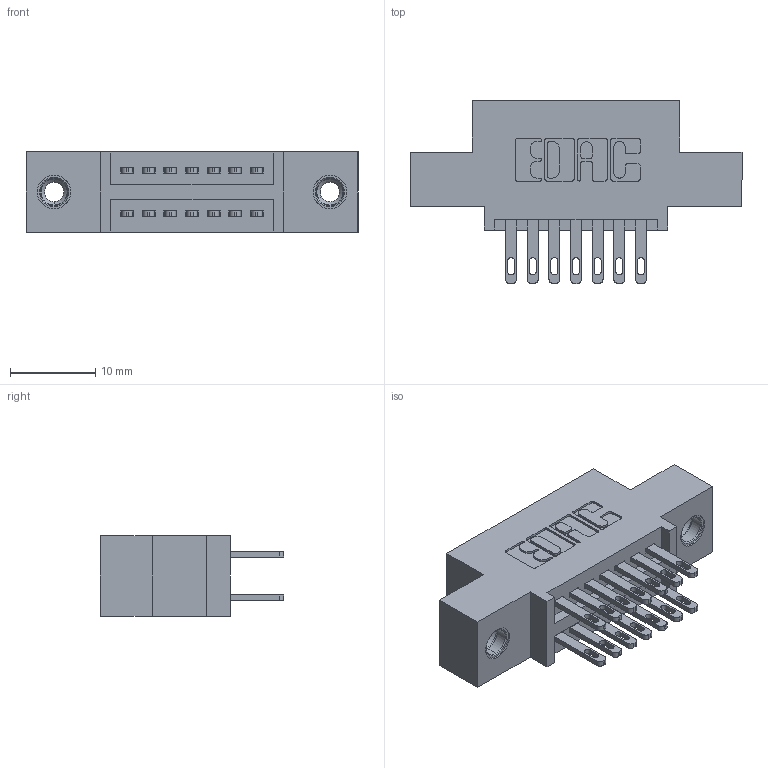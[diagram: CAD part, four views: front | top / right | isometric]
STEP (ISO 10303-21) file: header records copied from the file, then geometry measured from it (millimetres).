
FILE_DESCRIPTION (( 'STEP AP203' ), '1' );
FILE_NAME ('345-014-500-508.STEP', '2018-08-18T07:43:23', ( '' ), ( '' ), 'SwSTEP 2.0', 'SolidWorks 2016', '' );
FILE_SCHEMA (( 'CONFIG_CONTROL_DESIGN' ));
Length unit declared in the file: inch
Products named in the file (4): 345-292-001_345-293-100; 345-250-001_345-250-003-102; 345-014-500-508; 345 Part_0.110 Offset - 0.156 Dia-TI
Assembly tree (17 placements, depth 2):
  345-014-500-508
    345 Part_0.110 Offset - 0.156 Dia-TI
    345-292-001_345-293-100  x14
    345-250-001_345-250-003-102  x2
Bounding box: 38.99 x 21.51 x 9.4 mm (x, y, z)
Volume: 3425.4 mm3; surface area: 4634.6 mm2
Topology: 17 solids, 17 shells, 834 faces, 2463 edges, 1634 vertices
Faces by surface type: plane 494, cylinder 324, cone 12, torus 4
Entity records: 11452 total; most frequent: CARTESIAN_POINT 1935, ORIENTED_EDGE 1862, DIRECTION 1777, EDGE_CURVE 931, VECTOR 747, LINE 747, VERTEX_POINT 616, AXIS2_PLACEMENT_3D 515
